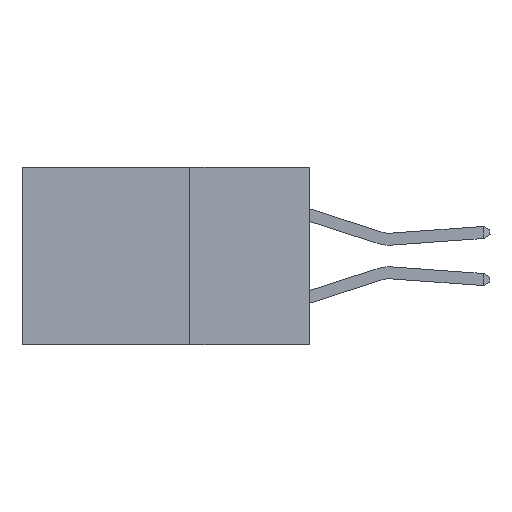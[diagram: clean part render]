
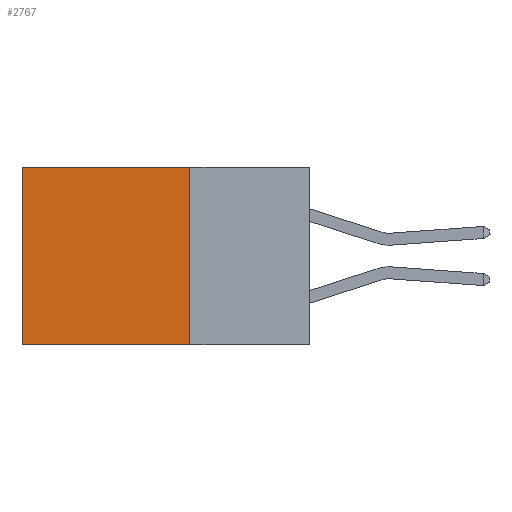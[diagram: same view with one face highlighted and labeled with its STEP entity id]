
A CAD part, left-side view. The second image highlights one B-rep face of the part: STEP entity #2767.
In plain terms, the highlighted planar face has unit normal (-1, 0, 0).
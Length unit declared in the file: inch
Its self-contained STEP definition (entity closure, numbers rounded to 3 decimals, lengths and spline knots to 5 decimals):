
#128 = LINE ( 'NONE', #8403, #2971 ) ;
#188 = DIRECTION ( 'NONE',  ( 0., 0., -1. ) ) ;
#547 = ORIENTED_EDGE ( 'NONE', *, *, #9644, .T. ) ;
#874 = EDGE_LOOP ( 'NONE', ( #547, #5172, #2402, #11050 ) ) ;
#953 = VERTEX_POINT ( 'NONE', #6137 ) ;
#1042 = LINE ( 'NONE', #4461, #10040 ) ;
#1506 = FACE_OUTER_BOUND ( 'NONE', #874, .T. ) ;
#1926 = VERTEX_POINT ( 'NONE', #7512 ) ;
#2402 = ORIENTED_EDGE ( 'NONE', *, *, #9162, .F. ) ;
#2767 = ADVANCED_FACE ( 'NONE', ( #1506 ), #9843, .F. ) ;
#2971 = VECTOR ( 'NONE', #188, 39.37008 ) ;
#3702 = DIRECTION ( 'NONE',  ( 0., 0., -1. ) ) ;
#4328 = VECTOR ( 'NONE', #6972, 39.37008 ) ;
#4448 = CARTESIAN_POINT ( 'NONE',  ( 0.2615, 0.25, -0.37 ) ) ;
#4461 = CARTESIAN_POINT ( 'NONE',  ( 0.2615, 0.25, -0.37 ) ) ;
#4622 = CARTESIAN_POINT ( 'NONE',  ( 0.2615, 0.6, -0.37 ) ) ;
#4702 = DIRECTION ( 'NONE',  ( 0., 1., 0. ) ) ;
#4780 = LINE ( 'NONE', #10404, #4328 ) ;
#5172 = ORIENTED_EDGE ( 'NONE', *, *, #8094, .F. ) ;
#5672 = VECTOR ( 'NONE', #3702, 39.37008 ) ;
#6137 = CARTESIAN_POINT ( 'NONE',  ( 0.2615, 0.6, 0. ) ) ;
#6311 = CARTESIAN_POINT ( 'NONE',  ( 0.2615, 0.6, -0.37 ) ) ;
#6933 = VERTEX_POINT ( 'NONE', #6311 ) ;
#6972 = DIRECTION ( 'NONE',  ( 0., 1., 0. ) ) ;
#7512 = CARTESIAN_POINT ( 'NONE',  ( 0.2615, 0.25, -0.37 ) ) ;
#8094 = EDGE_CURVE ( 'NONE', #1926, #6933, #1042, .T. ) ;
#8403 = CARTESIAN_POINT ( 'NONE',  ( 0.2615, 0.25, -0.37 ) ) ;
#8689 = CARTESIAN_POINT ( 'NONE',  ( 0.2615, 0.25, 0. ) ) ;
#9162 = EDGE_CURVE ( 'NONE', #11034, #1926, #128, .T. ) ;
#9338 = AXIS2_PLACEMENT_3D ( 'NONE', #4448, #11723, #11781 ) ;
#9644 = EDGE_CURVE ( 'NONE', #953, #6933, #11042, .T. ) ;
#9843 = PLANE ( 'NONE',  #9338 ) ;
#10040 = VECTOR ( 'NONE', #4702, 39.37008 ) ;
#10404 = CARTESIAN_POINT ( 'NONE',  ( 0.2615, 0.25, 0. ) ) ;
#10585 = EDGE_CURVE ( 'NONE', #11034, #953, #4780, .T. ) ;
#11034 = VERTEX_POINT ( 'NONE', #8689 ) ;
#11042 = LINE ( 'NONE', #4622, #5672 ) ;
#11050 = ORIENTED_EDGE ( 'NONE', *, *, #10585, .T. ) ;
#11723 = DIRECTION ( 'NONE',  ( 1., 0., 0. ) ) ;
#11781 = DIRECTION ( 'NONE',  ( 0., 0., -1. ) ) ;
